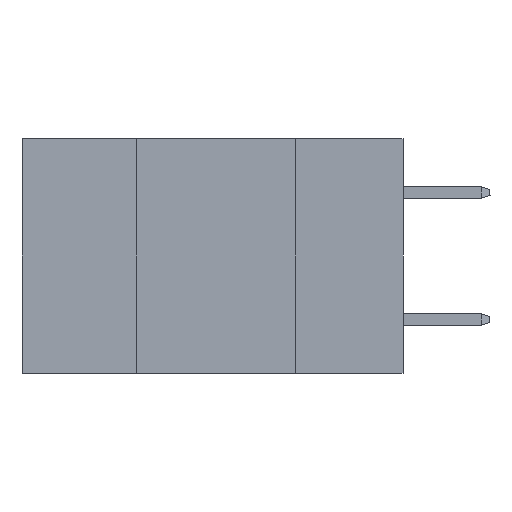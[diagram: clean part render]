
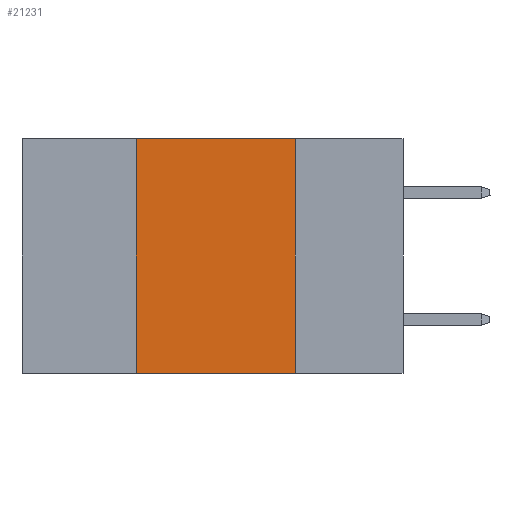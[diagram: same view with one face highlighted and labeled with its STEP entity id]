
A CAD part, left-side view. The second image highlights one B-rep face of the part: STEP entity #21231.
In plain terms, the highlighted planar face has unit normal (-1, 0, 0).
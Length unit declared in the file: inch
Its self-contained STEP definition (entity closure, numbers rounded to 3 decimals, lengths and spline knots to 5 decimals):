
#272 = CARTESIAN_POINT ( 'NONE',  ( 0., 0.42, -0.37 ) ) ;
#869 = CARTESIAN_POINT ( 'NONE',  ( 0., 0.17, -0.37 ) ) ;
#1655 = LINE ( 'NONE', #8086, #40517 ) ;
#1889 = DIRECTION ( 'NONE',  ( 0., 0., 1. ) ) ;
#2090 = CARTESIAN_POINT ( 'NONE',  ( 0., 0.6, 0. ) ) ;
#2796 = DIRECTION ( 'NONE',  ( 0., -1., 0. ) ) ;
#3092 = CARTESIAN_POINT ( 'NONE',  ( 0., 0.6, 0. ) ) ;
#3515 = ORIENTED_EDGE ( 'NONE', *, *, #8044, .F. ) ;
#6014 = EDGE_CURVE ( 'NONE', #36959, #19544, #39055, .T. ) ;
#8044 = EDGE_CURVE ( 'NONE', #36959, #14537, #1655, .T. ) ;
#8086 = CARTESIAN_POINT ( 'NONE',  ( 0., 0.42, 0. ) ) ;
#9985 = PLANE ( 'NONE',  #40112 ) ;
#10667 = EDGE_CURVE ( 'NONE', #14537, #21790, #20116, .T. ) ;
#13540 = DIRECTION ( 'NONE',  ( 0., -1., 0. ) ) ;
#14537 = VERTEX_POINT ( 'NONE', #28153 ) ;
#17588 = DIRECTION ( 'NONE',  ( 0., 0., -1. ) ) ;
#19544 = VERTEX_POINT ( 'NONE', #869 ) ;
#20116 = LINE ( 'NONE', #2090, #43577 ) ;
#21231 = ADVANCED_FACE ( 'NONE', ( #35060 ), #9985, .F. ) ;
#21790 = VERTEX_POINT ( 'NONE', #24363 ) ;
#24363 = CARTESIAN_POINT ( 'NONE',  ( 0., 0.17, 0. ) ) ;
#25503 = EDGE_CURVE ( 'NONE', #21790, #19544, #35383, .T. ) ;
#26849 = VECTOR ( 'NONE', #13540, 39.37008 ) ;
#28153 = CARTESIAN_POINT ( 'NONE',  ( 0., 0.42, 0. ) ) ;
#30810 = CARTESIAN_POINT ( 'NONE',  ( 0., 0.6, -0.37 ) ) ;
#32435 = ORIENTED_EDGE ( 'NONE', *, *, #10667, .F. ) ;
#33569 = ORIENTED_EDGE ( 'NONE', *, *, #6014, .T. ) ;
#34226 = VECTOR ( 'NONE', #38690, 39.37008 ) ;
#35060 = FACE_OUTER_BOUND ( 'NONE', #37676, .T. ) ;
#35383 = LINE ( 'NONE', #46243, #34226 ) ;
#36959 = VERTEX_POINT ( 'NONE', #272 ) ;
#37676 = EDGE_LOOP ( 'NONE', ( #42308, #32435, #3515, #33569 ) ) ;
#38690 = DIRECTION ( 'NONE',  ( 0., 0., -1. ) ) ;
#39055 = LINE ( 'NONE', #30810, #26849 ) ;
#40112 = AXIS2_PLACEMENT_3D ( 'NONE', #3092, #44562, #17588 ) ;
#40517 = VECTOR ( 'NONE', #1889, 39.37008 ) ;
#42308 = ORIENTED_EDGE ( 'NONE', *, *, #25503, .F. ) ;
#43577 = VECTOR ( 'NONE', #2796, 39.37008 ) ;
#44562 = DIRECTION ( 'NONE',  ( 1., 0., 0. ) ) ;
#46243 = CARTESIAN_POINT ( 'NONE',  ( 0., 0.17, 0. ) ) ;
